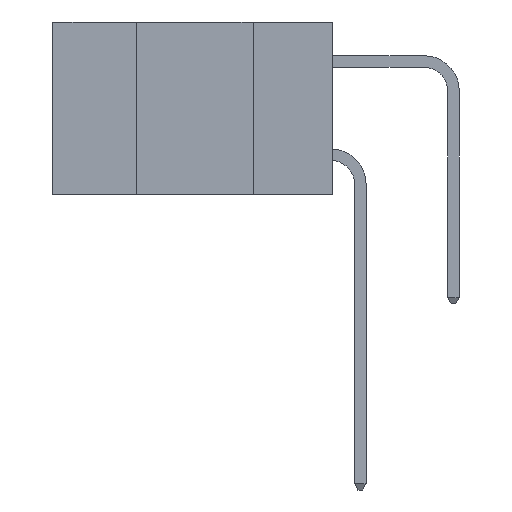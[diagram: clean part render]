
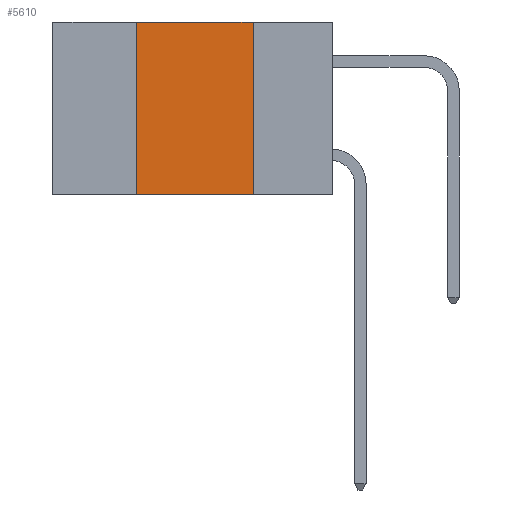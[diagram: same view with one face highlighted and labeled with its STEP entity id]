
A CAD part, left-side view. The second image highlights one B-rep face of the part: STEP entity #5610.
In plain terms, the highlighted planar face has unit normal (-1, 0, 0).
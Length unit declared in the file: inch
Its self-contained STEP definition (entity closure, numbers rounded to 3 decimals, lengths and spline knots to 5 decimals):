
#228 = LINE ( 'NONE', #5706, #5111 ) ;
#453 = LINE ( 'NONE', #11578, #3088 ) ;
#493 = EDGE_CURVE ( 'NONE', #2279, #2337, #6140, .T. ) ;
#513 = CARTESIAN_POINT ( 'NONE',  ( 0., 0.42, -0.37 ) ) ;
#1919 = PLANE ( 'NONE',  #9081 ) ;
#2052 = DIRECTION ( 'NONE',  ( 0., 0., -1. ) ) ;
#2158 = DIRECTION ( 'NONE',  ( 0., 0., 1. ) ) ;
#2279 = VERTEX_POINT ( 'NONE', #4777 ) ;
#2337 = VERTEX_POINT ( 'NONE', #3606 ) ;
#2699 = FACE_OUTER_BOUND ( 'NONE', #5295, .T. ) ;
#3088 = VECTOR ( 'NONE', #12503, 39.37008 ) ;
#3606 = CARTESIAN_POINT ( 'NONE',  ( 0., 0.17, -0.37 ) ) ;
#3996 = CARTESIAN_POINT ( 'NONE',  ( 0., 0.6, 0. ) ) ;
#4596 = ORIENTED_EDGE ( 'NONE', *, *, #10025, .T. ) ;
#4777 = CARTESIAN_POINT ( 'NONE',  ( 0., 0.17, 0. ) ) ;
#5111 = VECTOR ( 'NONE', #11481, 39.37008 ) ;
#5295 = EDGE_LOOP ( 'NONE', ( #8224, #9131, #8723, #4596 ) ) ;
#5610 = ADVANCED_FACE ( 'NONE', ( #2699 ), #1919, .F. ) ;
#5706 = CARTESIAN_POINT ( 'NONE',  ( 0., 0.6, -0.37 ) ) ;
#6140 = LINE ( 'NONE', #8423, #11550 ) ;
#6892 = EDGE_CURVE ( 'NONE', #7502, #2279, #453, .T. ) ;
#7244 = VECTOR ( 'NONE', #2158, 39.37008 ) ;
#7502 = VERTEX_POINT ( 'NONE', #10743 ) ;
#7913 = DIRECTION ( 'NONE',  ( 1., 0., 0. ) ) ;
#8224 = ORIENTED_EDGE ( 'NONE', *, *, #493, .F. ) ;
#8423 = CARTESIAN_POINT ( 'NONE',  ( 0., 0.17, -0.37 ) ) ;
#8723 = ORIENTED_EDGE ( 'NONE', *, *, #9619, .F. ) ;
#9081 = AXIS2_PLACEMENT_3D ( 'NONE', #3996, #7913, #2052 ) ;
#9131 = ORIENTED_EDGE ( 'NONE', *, *, #6892, .F. ) ;
#9330 = DIRECTION ( 'NONE',  ( 0., 0., -1. ) ) ;
#9619 = EDGE_CURVE ( 'NONE', #9803, #7502, #9847, .T. ) ;
#9803 = VERTEX_POINT ( 'NONE', #513 ) ;
#9847 = LINE ( 'NONE', #9988, #7244 ) ;
#9988 = CARTESIAN_POINT ( 'NONE',  ( 0., 0.42, -0.37 ) ) ;
#10025 = EDGE_CURVE ( 'NONE', #9803, #2337, #228, .T. ) ;
#10743 = CARTESIAN_POINT ( 'NONE',  ( 0., 0.42, 0. ) ) ;
#11481 = DIRECTION ( 'NONE',  ( 0., -1., 0. ) ) ;
#11550 = VECTOR ( 'NONE', #9330, 39.37008 ) ;
#11578 = CARTESIAN_POINT ( 'NONE',  ( 0., 0.6, 0. ) ) ;
#12503 = DIRECTION ( 'NONE',  ( 0., -1., 0. ) ) ;
